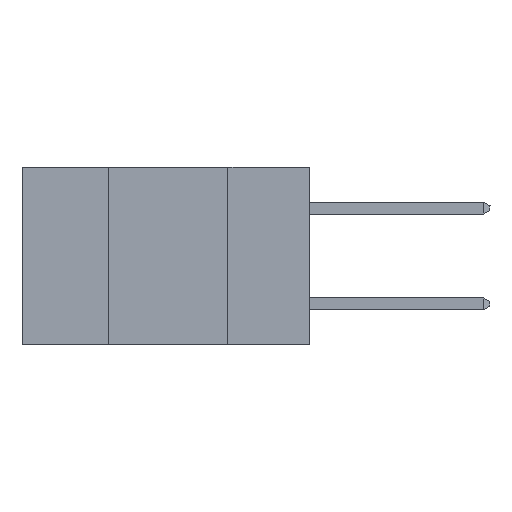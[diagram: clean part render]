
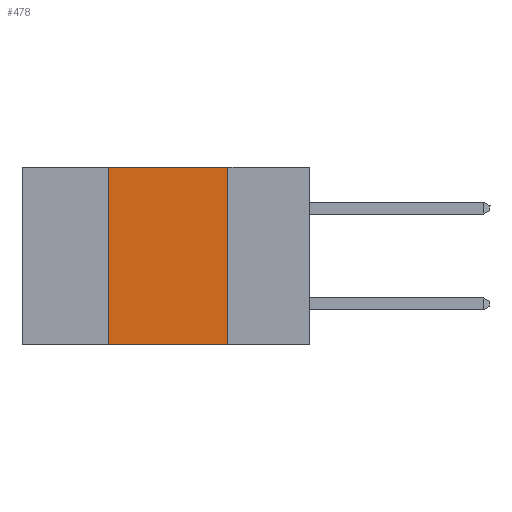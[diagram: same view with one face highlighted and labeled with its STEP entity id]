
A CAD part, left-side view. The second image highlights one B-rep face of the part: STEP entity #478.
In plain terms, the highlighted planar face has unit normal (-1, 0, 0).
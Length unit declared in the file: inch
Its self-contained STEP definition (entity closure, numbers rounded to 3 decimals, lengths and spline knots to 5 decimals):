
#46 = LINE ( 'NONE', #9873, #15517 ) ;
#478 = ADVANCED_FACE ( 'NONE', ( #16955 ), #14957, .F. ) ;
#719 = CARTESIAN_POINT ( 'NONE',  ( 0., 0.6, 0. ) ) ;
#2306 = LINE ( 'NONE', #13934, #14035 ) ;
#2500 = ORIENTED_EDGE ( 'NONE', *, *, #11221, .F. ) ;
#3965 = CARTESIAN_POINT ( 'NONE',  ( 0., 0.17, -0.37 ) ) ;
#3969 = DIRECTION ( 'NONE',  ( 0., 0., 1. ) ) ;
#4061 = VECTOR ( 'NONE', #5739, 39.37008 ) ;
#4144 = EDGE_CURVE ( 'NONE', #9798, #14114, #4515, .T. ) ;
#4515 = LINE ( 'NONE', #14298, #4061 ) ;
#4706 = EDGE_CURVE ( 'NONE', #9798, #18864, #46, .T. ) ;
#5143 = EDGE_CURVE ( 'NONE', #18864, #16416, #17879, .T. ) ;
#5364 = ORIENTED_EDGE ( 'NONE', *, *, #5143, .F. ) ;
#5739 = DIRECTION ( 'NONE',  ( 0., -1., 0. ) ) ;
#6576 = EDGE_LOOP ( 'NONE', ( #2500, #5364, #8273, #9161 ) ) ;
#6762 = DIRECTION ( 'NONE',  ( 0., -1., 0. ) ) ;
#8273 = ORIENTED_EDGE ( 'NONE', *, *, #4706, .F. ) ;
#9161 = ORIENTED_EDGE ( 'NONE', *, *, #4144, .T. ) ;
#9798 = VERTEX_POINT ( 'NONE', #12294 ) ;
#9873 = CARTESIAN_POINT ( 'NONE',  ( 0., 0.42, 0. ) ) ;
#10149 = AXIS2_PLACEMENT_3D ( 'NONE', #13402, #14892, #10740 ) ;
#10740 = DIRECTION ( 'NONE',  ( 0., 0., -1. ) ) ;
#11221 = EDGE_CURVE ( 'NONE', #16416, #14114, #2306, .T. ) ;
#12294 = CARTESIAN_POINT ( 'NONE',  ( 0., 0.42, -0.37 ) ) ;
#13402 = CARTESIAN_POINT ( 'NONE',  ( 0., 0.6, 0. ) ) ;
#13816 = DIRECTION ( 'NONE',  ( 0., 0., -1. ) ) ;
#13934 = CARTESIAN_POINT ( 'NONE',  ( 0., 0.17, 0. ) ) ;
#14035 = VECTOR ( 'NONE', #13816, 39.37008 ) ;
#14114 = VERTEX_POINT ( 'NONE', #3965 ) ;
#14202 = CARTESIAN_POINT ( 'NONE',  ( 0., 0.42, 0. ) ) ;
#14298 = CARTESIAN_POINT ( 'NONE',  ( 0., 0.6, -0.37 ) ) ;
#14338 = VECTOR ( 'NONE', #6762, 39.37008 ) ;
#14892 = DIRECTION ( 'NONE',  ( 1., 0., 0. ) ) ;
#14957 = PLANE ( 'NONE',  #10149 ) ;
#15517 = VECTOR ( 'NONE', #3969, 39.37008 ) ;
#16416 = VERTEX_POINT ( 'NONE', #17478 ) ;
#16955 = FACE_OUTER_BOUND ( 'NONE', #6576, .T. ) ;
#17478 = CARTESIAN_POINT ( 'NONE',  ( 0., 0.17, 0. ) ) ;
#17879 = LINE ( 'NONE', #719, #14338 ) ;
#18864 = VERTEX_POINT ( 'NONE', #14202 ) ;
